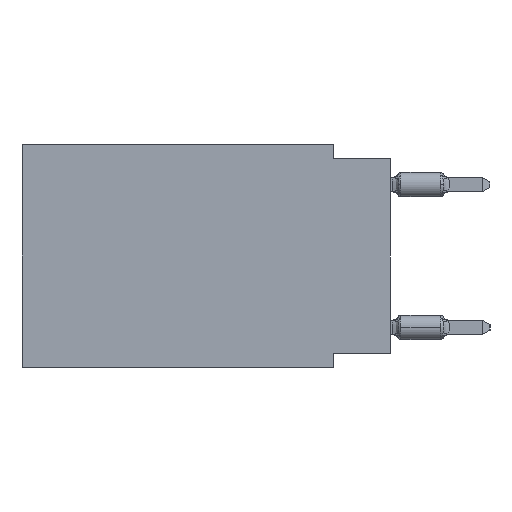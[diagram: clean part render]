
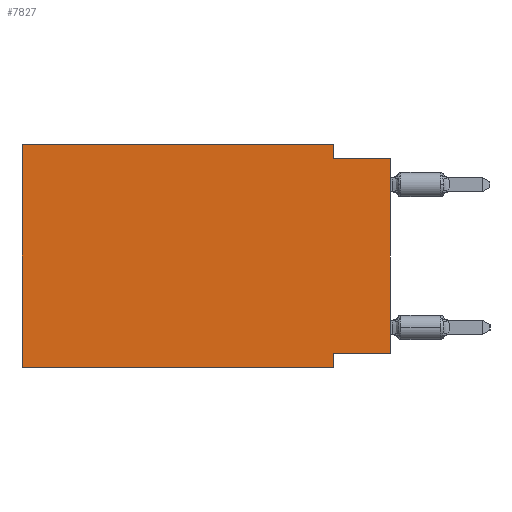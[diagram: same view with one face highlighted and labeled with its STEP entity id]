
A CAD part, left-side view. The second image highlights one B-rep face of the part: STEP entity #7827.
In plain terms, the highlighted planar face has unit normal (-1, 0, 0).
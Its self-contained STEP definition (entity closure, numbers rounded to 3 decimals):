
#2020 = DIRECTION ( 'NONE',  ( 0., 0., -1. ) ) ;
#2395 = EDGE_CURVE ( 'NONE', #63296, #19296, #31072, .T. ) ;
#2570 = EDGE_CURVE ( 'NONE', #4509, #62048, #43122, .T. ) ;
#3241 = DIRECTION ( 'NONE',  ( 0., -1., 0. ) ) ;
#3298 = EDGE_CURVE ( 'NONE', #60371, #19296, #6133, .T. ) ;
#3497 = VERTEX_POINT ( 'NONE', #61580 ) ;
#3932 = VECTOR ( 'NONE', #3241, 1000. ) ;
#4293 = EDGE_CURVE ( 'NONE', #31403, #27254, #4457, .T. ) ;
#4457 = LINE ( 'NONE', #36244, #53240 ) ;
#4509 = VERTEX_POINT ( 'NONE', #42599 ) ;
#6133 = LINE ( 'NONE', #21896, #48945 ) ;
#7080 = ORIENTED_EDGE ( 'NONE', *, *, #2570, .F. ) ;
#7116 = DIRECTION ( 'NONE',  ( 0., 0., -1. ) ) ;
#7715 = PLANE ( 'NONE',  #39683 ) ;
#7827 = ADVANCED_FACE ( 'NONE', ( #27479 ), #7715, .F. ) ;
#7955 = CARTESIAN_POINT ( 'NONE',  ( 0., 0., -0.635 ) ) ;
#12099 = CARTESIAN_POINT ( 'NONE',  ( 0., 2.54, -9.271 ) ) ;
#15427 = VECTOR ( 'NONE', #57960, 1000. ) ;
#15492 = DIRECTION ( 'NONE',  ( 0., -1., 0. ) ) ;
#16444 = VECTOR ( 'NONE', #54575, 1000. ) ;
#16748 = VECTOR ( 'NONE', #57867, 1000. ) ;
#17011 = CARTESIAN_POINT ( 'NONE',  ( 0., 16.383, -9.906 ) ) ;
#17209 = ORIENTED_EDGE ( 'NONE', *, *, #39626, .F. ) ;
#17445 = DIRECTION ( 'NONE',  ( 1., 0., 0. ) ) ;
#19296 = VERTEX_POINT ( 'NONE', #19966 ) ;
#19966 = CARTESIAN_POINT ( 'NONE',  ( 0., 2.54, -9.906 ) ) ;
#21896 = CARTESIAN_POINT ( 'NONE',  ( 0., 2.54, -9.906 ) ) ;
#22084 = EDGE_LOOP ( 'NONE', ( #56417, #7080, #17209, #48140, #65937, #23201, #40661, #54303 ) ) ;
#23201 = ORIENTED_EDGE ( 'NONE', *, *, #2395, .T. ) ;
#26417 = CARTESIAN_POINT ( 'NONE',  ( 0., 0., -9.271 ) ) ;
#26468 = EDGE_CURVE ( 'NONE', #3497, #60371, #30453, .T. ) ;
#27143 = CARTESIAN_POINT ( 'NONE',  ( 0., 0., 0. ) ) ;
#27254 = VERTEX_POINT ( 'NONE', #54446 ) ;
#27479 = FACE_OUTER_BOUND ( 'NONE', #22084, .T. ) ;
#30453 = LINE ( 'NONE', #26417, #38870 ) ;
#30593 = DIRECTION ( 'NONE',  ( 0., 0., -1. ) ) ;
#31072 = LINE ( 'NONE', #17011, #16748 ) ;
#31403 = VERTEX_POINT ( 'NONE', #59482 ) ;
#32577 = LINE ( 'NONE', #53018, #41618 ) ;
#36244 = CARTESIAN_POINT ( 'NONE',  ( 0., 16.383, 0. ) ) ;
#37865 = LINE ( 'NONE', #27143, #15427 ) ;
#38870 = VECTOR ( 'NONE', #62254, 1000. ) ;
#39489 = LINE ( 'NONE', #49555, #16444 ) ;
#39626 = EDGE_CURVE ( 'NONE', #27254, #4509, #32577, .T. ) ;
#39683 = AXIS2_PLACEMENT_3D ( 'NONE', #63336, #17445, #2020 ) ;
#40661 = ORIENTED_EDGE ( 'NONE', *, *, #3298, .F. ) ;
#41618 = VECTOR ( 'NONE', #7116, 1000. ) ;
#42599 = CARTESIAN_POINT ( 'NONE',  ( 0., 2.54, -0.635 ) ) ;
#43122 = LINE ( 'NONE', #7955, #3932 ) ;
#48140 = ORIENTED_EDGE ( 'NONE', *, *, #4293, .F. ) ;
#48945 = VECTOR ( 'NONE', #30593, 1000. ) ;
#49555 = CARTESIAN_POINT ( 'NONE',  ( 0., 16.383, 0. ) ) ;
#52334 = CARTESIAN_POINT ( 'NONE',  ( 0., 16.383, -9.906 ) ) ;
#53018 = CARTESIAN_POINT ( 'NONE',  ( 0., 2.54, 0. ) ) ;
#53240 = VECTOR ( 'NONE', #15492, 1000. ) ;
#54303 = ORIENTED_EDGE ( 'NONE', *, *, #26468, .F. ) ;
#54446 = CARTESIAN_POINT ( 'NONE',  ( 0., 2.54, 0. ) ) ;
#54575 = DIRECTION ( 'NONE',  ( 0., 0., 1. ) ) ;
#54958 = EDGE_CURVE ( 'NONE', #63296, #31403, #39489, .T. ) ;
#56417 = ORIENTED_EDGE ( 'NONE', *, *, #57895, .T. ) ;
#57867 = DIRECTION ( 'NONE',  ( 0., -1., 0. ) ) ;
#57895 = EDGE_CURVE ( 'NONE', #3497, #62048, #37865, .T. ) ;
#57960 = DIRECTION ( 'NONE',  ( 0., 0., 1. ) ) ;
#59482 = CARTESIAN_POINT ( 'NONE',  ( 0., 16.383, 0. ) ) ;
#60371 = VERTEX_POINT ( 'NONE', #12099 ) ;
#61580 = CARTESIAN_POINT ( 'NONE',  ( 0., 0., -9.271 ) ) ;
#62048 = VERTEX_POINT ( 'NONE', #63639 ) ;
#62254 = DIRECTION ( 'NONE',  ( 0., 1., 0. ) ) ;
#63296 = VERTEX_POINT ( 'NONE', #52334 ) ;
#63336 = CARTESIAN_POINT ( 'NONE',  ( 0., 16.383, 0. ) ) ;
#63639 = CARTESIAN_POINT ( 'NONE',  ( 0., 0., -0.635 ) ) ;
#65937 = ORIENTED_EDGE ( 'NONE', *, *, #54958, .F. ) ;
